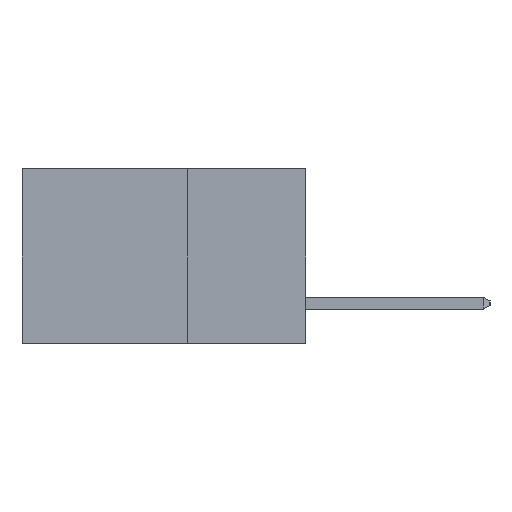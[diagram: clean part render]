
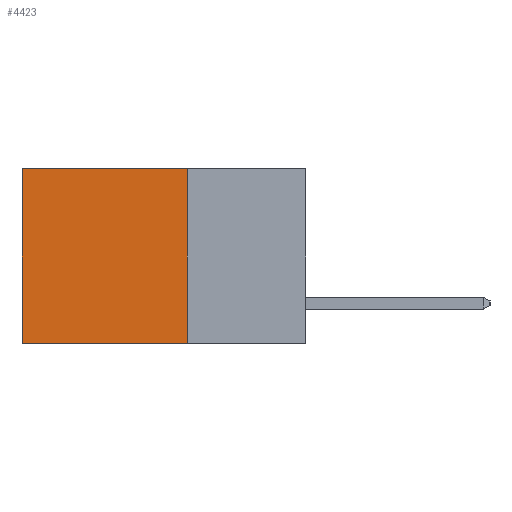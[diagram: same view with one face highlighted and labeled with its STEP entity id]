
A CAD part, left-side view. The second image highlights one B-rep face of the part: STEP entity #4423.
In plain terms, the highlighted planar face has unit normal (-1, 0, 0).
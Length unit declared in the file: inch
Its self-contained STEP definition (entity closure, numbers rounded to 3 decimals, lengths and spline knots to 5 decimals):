
#126 = ORIENTED_EDGE ( 'NONE', *, *, #11208, .F. ) ;
#310 = VECTOR ( 'NONE', #8097, 39.37008 ) ;
#897 = EDGE_CURVE ( 'NONE', #13738, #1266, #14299, .T. ) ;
#1266 = VERTEX_POINT ( 'NONE', #2606 ) ;
#1539 = DIRECTION ( 'NONE',  ( 0., 0., -1. ) ) ;
#1563 = VECTOR ( 'NONE', #3052, 39.37008 ) ;
#1585 = DIRECTION ( 'NONE',  ( 1., 0., 0. ) ) ;
#1589 = PLANE ( 'NONE',  #7014 ) ;
#1709 = CARTESIAN_POINT ( 'NONE',  ( 0.2615, 0.25, -0.37 ) ) ;
#2017 = DIRECTION ( 'NONE',  ( 0., 0., -1. ) ) ;
#2168 = CARTESIAN_POINT ( 'NONE',  ( 0.2615, 0.25, -0.37 ) ) ;
#2406 = CARTESIAN_POINT ( 'NONE',  ( 0.2615, 0.25, 0. ) ) ;
#2487 = ORIENTED_EDGE ( 'NONE', *, *, #897, .T. ) ;
#2606 = CARTESIAN_POINT ( 'NONE',  ( 0.2615, 0.6, 0. ) ) ;
#3052 = DIRECTION ( 'NONE',  ( 0., 1., 0. ) ) ;
#3098 = VERTEX_POINT ( 'NONE', #3932 ) ;
#3340 = VECTOR ( 'NONE', #2017, 39.37008 ) ;
#3341 = VERTEX_POINT ( 'NONE', #2168 ) ;
#3932 = CARTESIAN_POINT ( 'NONE',  ( 0.2615, 0.6, -0.37 ) ) ;
#4423 = ADVANCED_FACE ( 'NONE', ( #8319 ), #1589, .F. ) ;
#4480 = ORIENTED_EDGE ( 'NONE', *, *, #11783, .F. ) ;
#6000 = CARTESIAN_POINT ( 'NONE',  ( 0.2615, 0.25, 0. ) ) ;
#6004 = ORIENTED_EDGE ( 'NONE', *, *, #12639, .T. ) ;
#6017 = DIRECTION ( 'NONE',  ( 0., 1., 0. ) ) ;
#6961 = CARTESIAN_POINT ( 'NONE',  ( 0.2615, 0.6, -0.37 ) ) ;
#7014 = AXIS2_PLACEMENT_3D ( 'NONE', #1709, #1585, #1539 ) ;
#8097 = DIRECTION ( 'NONE',  ( 0., 0., -1. ) ) ;
#8319 = FACE_OUTER_BOUND ( 'NONE', #12668, .T. ) ;
#8592 = VECTOR ( 'NONE', #6017, 39.37008 ) ;
#9842 = CARTESIAN_POINT ( 'NONE',  ( 0.2615, 0.25, -0.37 ) ) ;
#10230 = LINE ( 'NONE', #9842, #1563 ) ;
#11062 = CARTESIAN_POINT ( 'NONE',  ( 0.2615, 0.25, -0.37 ) ) ;
#11208 = EDGE_CURVE ( 'NONE', #13738, #3341, #12282, .T. ) ;
#11783 = EDGE_CURVE ( 'NONE', #3341, #3098, #10230, .T. ) ;
#11930 = LINE ( 'NONE', #6961, #310 ) ;
#12282 = LINE ( 'NONE', #11062, #3340 ) ;
#12639 = EDGE_CURVE ( 'NONE', #1266, #3098, #11930, .T. ) ;
#12668 = EDGE_LOOP ( 'NONE', ( #6004, #4480, #126, #2487 ) ) ;
#13738 = VERTEX_POINT ( 'NONE', #2406 ) ;
#14299 = LINE ( 'NONE', #6000, #8592 ) ;
